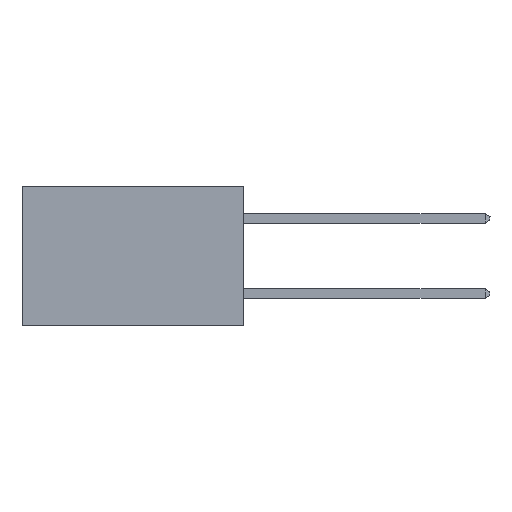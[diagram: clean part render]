
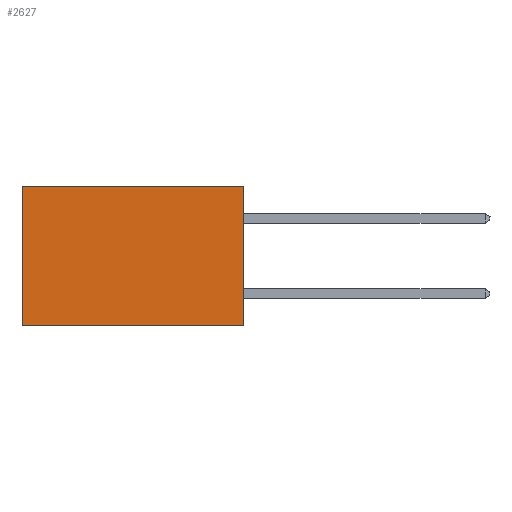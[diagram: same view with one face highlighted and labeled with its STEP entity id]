
A CAD part, left-side view. The second image highlights one B-rep face of the part: STEP entity #2627.
In plain terms, the highlighted planar face has unit normal (-1, 0, 0).
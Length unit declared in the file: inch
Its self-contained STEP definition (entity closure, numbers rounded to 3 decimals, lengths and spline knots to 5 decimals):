
#1027 = ORIENTED_EDGE ( 'NONE', *, *, #17807, .F. ) ;
#1259 = CARTESIAN_POINT ( 'NONE',  ( 0.277, 0.59, 0. ) ) ;
#1680 = ORIENTED_EDGE ( 'NONE', *, *, #14088, .T. ) ;
#2627 = ADVANCED_FACE ( 'NONE', ( #22684 ), #20957, .F. ) ;
#3020 = CARTESIAN_POINT ( 'NONE',  ( 0.277, 0., 0. ) ) ;
#4705 = VECTOR ( 'NONE', #22634, 39.37008 ) ;
#6763 = CARTESIAN_POINT ( 'NONE',  ( 0.277, 0., 0. ) ) ;
#6878 = CARTESIAN_POINT ( 'NONE',  ( 0.277, 0., -0.37 ) ) ;
#7435 = VERTEX_POINT ( 'NONE', #3020 ) ;
#7753 = EDGE_CURVE ( 'NONE', #15348, #26854, #31120, .T. ) ;
#8031 = DIRECTION ( 'NONE',  ( 0., 0., -1. ) ) ;
#9556 = DIRECTION ( 'NONE',  ( 0., 1., 0. ) ) ;
#9939 = VECTOR ( 'NONE', #9556, 39.37008 ) ;
#12362 = CARTESIAN_POINT ( 'NONE',  ( 0.277, 0., -0.37 ) ) ;
#14088 = EDGE_CURVE ( 'NONE', #7435, #19850, #18790, .T. ) ;
#14997 = DIRECTION ( 'NONE',  ( 0., 0., -1. ) ) ;
#15348 = VERTEX_POINT ( 'NONE', #19901 ) ;
#15613 = DIRECTION ( 'NONE',  ( 0., 0., -1. ) ) ;
#16072 = ORIENTED_EDGE ( 'NONE', *, *, #26246, .T. ) ;
#16492 = VECTOR ( 'NONE', #8031, 39.37008 ) ;
#17807 = EDGE_CURVE ( 'NONE', #7435, #15348, #33959, .T. ) ;
#18790 = LINE ( 'NONE', #6763, #4705 ) ;
#18978 = VECTOR ( 'NONE', #14997, 39.37008 ) ;
#19530 = ORIENTED_EDGE ( 'NONE', *, *, #7753, .F. ) ;
#19850 = VERTEX_POINT ( 'NONE', #1259 ) ;
#19901 = CARTESIAN_POINT ( 'NONE',  ( 0.277, 0., -0.37 ) ) ;
#20297 = DIRECTION ( 'NONE',  ( 1., 0., 0. ) ) ;
#20957 = PLANE ( 'NONE',  #26293 ) ;
#21237 = CARTESIAN_POINT ( 'NONE',  ( 0.277, 0.59, -0.37 ) ) ;
#22634 = DIRECTION ( 'NONE',  ( 0., 1., 0. ) ) ;
#22684 = FACE_OUTER_BOUND ( 'NONE', #33384, .T. ) ;
#23516 = CARTESIAN_POINT ( 'NONE',  ( 0.277, 0.59, -0.37 ) ) ;
#23625 = CARTESIAN_POINT ( 'NONE',  ( 0.277, 0., -0.37 ) ) ;
#26246 = EDGE_CURVE ( 'NONE', #19850, #26854, #30669, .T. ) ;
#26293 = AXIS2_PLACEMENT_3D ( 'NONE', #23625, #20297, #15613 ) ;
#26854 = VERTEX_POINT ( 'NONE', #23516 ) ;
#30669 = LINE ( 'NONE', #21237, #16492 ) ;
#31120 = LINE ( 'NONE', #6878, #9939 ) ;
#33384 = EDGE_LOOP ( 'NONE', ( #16072, #19530, #1027, #1680 ) ) ;
#33959 = LINE ( 'NONE', #12362, #18978 ) ;
